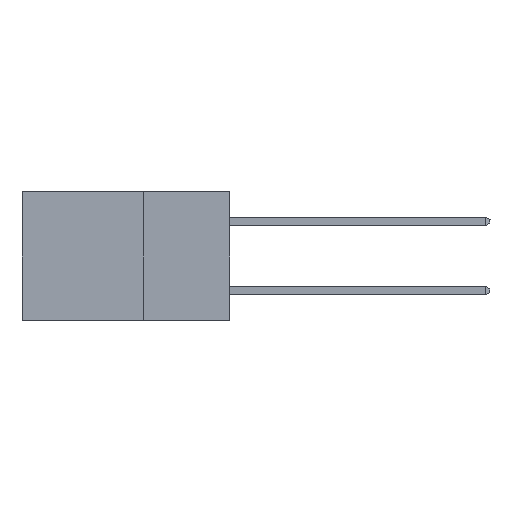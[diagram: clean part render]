
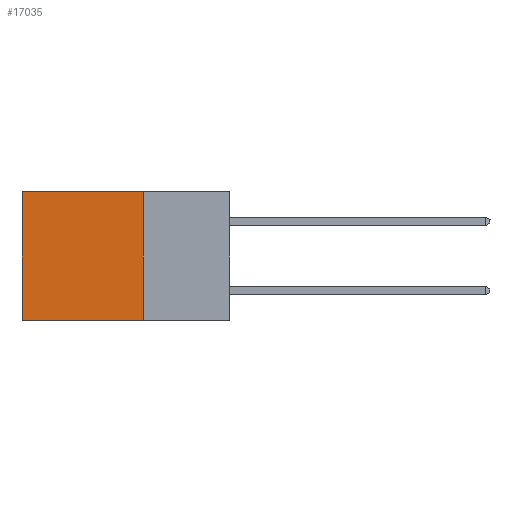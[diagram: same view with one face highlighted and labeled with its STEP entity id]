
A CAD part, left-side view. The second image highlights one B-rep face of the part: STEP entity #17035.
In plain terms, the highlighted planar face has unit normal (-1, 0, 0).
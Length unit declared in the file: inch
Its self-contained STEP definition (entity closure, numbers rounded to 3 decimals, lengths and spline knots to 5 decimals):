
#1325 = VERTEX_POINT ( 'NONE', #16195 ) ;
#1719 = VECTOR ( 'NONE', #1795, 39.37008 ) ;
#1795 = DIRECTION ( 'NONE',  ( 0., 0., -1. ) ) ;
#2515 = LINE ( 'NONE', #11906, #12065 ) ;
#2548 = ORIENTED_EDGE ( 'NONE', *, *, #6720, .T. ) ;
#2691 = DIRECTION ( 'NONE',  ( 0., 0., -1. ) ) ;
#3012 = CARTESIAN_POINT ( 'NONE',  ( 0.2615, 0.6, -0.37 ) ) ;
#3109 = EDGE_CURVE ( 'NONE', #1325, #6336, #2515, .T. ) ;
#4231 = CARTESIAN_POINT ( 'NONE',  ( 0.2615, 0.6, 0. ) ) ;
#4370 = EDGE_CURVE ( 'NONE', #1325, #14877, #15766, .T. ) ;
#4433 = CARTESIAN_POINT ( 'NONE',  ( 0.2615, 0.25, -0.37 ) ) ;
#4484 = ORIENTED_EDGE ( 'NONE', *, *, #3109, .F. ) ;
#5320 = FACE_OUTER_BOUND ( 'NONE', #10189, .T. ) ;
#5685 = ORIENTED_EDGE ( 'NONE', *, *, #4370, .T. ) ;
#5920 = PLANE ( 'NONE',  #11227 ) ;
#6336 = VERTEX_POINT ( 'NONE', #4433 ) ;
#6720 = EDGE_CURVE ( 'NONE', #14877, #7382, #6951, .T. ) ;
#6951 = LINE ( 'NONE', #3012, #1719 ) ;
#7382 = VERTEX_POINT ( 'NONE', #9107 ) ;
#7976 = LINE ( 'NONE', #14542, #13425 ) ;
#8035 = DIRECTION ( 'NONE',  ( 1., 0., 0. ) ) ;
#8246 = DIRECTION ( 'NONE',  ( 0., 1., 0. ) ) ;
#9107 = CARTESIAN_POINT ( 'NONE',  ( 0.2615, 0.6, -0.37 ) ) ;
#10189 = EDGE_LOOP ( 'NONE', ( #2548, #16202, #4484, #5685 ) ) ;
#10241 = EDGE_CURVE ( 'NONE', #6336, #7382, #7976, .T. ) ;
#10666 = CARTESIAN_POINT ( 'NONE',  ( 0.2615, 0.25, 0. ) ) ;
#11227 = AXIS2_PLACEMENT_3D ( 'NONE', #13557, #8035, #2691 ) ;
#11906 = CARTESIAN_POINT ( 'NONE',  ( 0.2615, 0.25, -0.37 ) ) ;
#11975 = DIRECTION ( 'NONE',  ( 0., 1., 0. ) ) ;
#12065 = VECTOR ( 'NONE', #13292, 39.37008 ) ;
#12480 = VECTOR ( 'NONE', #11975, 39.37008 ) ;
#13292 = DIRECTION ( 'NONE',  ( 0., 0., -1. ) ) ;
#13425 = VECTOR ( 'NONE', #8246, 39.37008 ) ;
#13557 = CARTESIAN_POINT ( 'NONE',  ( 0.2615, 0.25, -0.37 ) ) ;
#14542 = CARTESIAN_POINT ( 'NONE',  ( 0.2615, 0.25, -0.37 ) ) ;
#14877 = VERTEX_POINT ( 'NONE', #4231 ) ;
#15766 = LINE ( 'NONE', #10666, #12480 ) ;
#16195 = CARTESIAN_POINT ( 'NONE',  ( 0.2615, 0.25, 0. ) ) ;
#16202 = ORIENTED_EDGE ( 'NONE', *, *, #10241, .F. ) ;
#17035 = ADVANCED_FACE ( 'NONE', ( #5320 ), #5920, .F. ) ;
